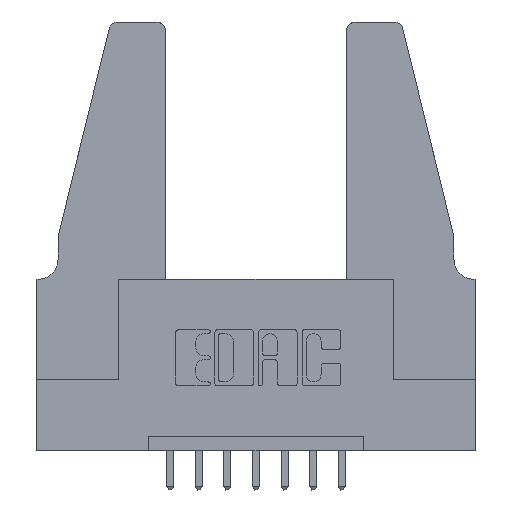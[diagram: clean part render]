
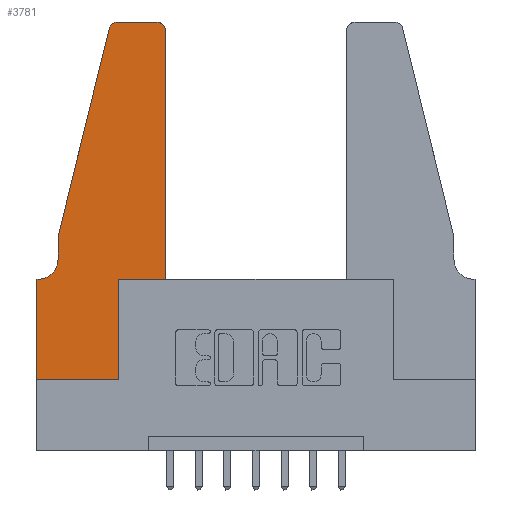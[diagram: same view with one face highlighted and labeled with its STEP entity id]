
A CAD part, top view. The second image highlights one B-rep face of the part: STEP entity #3781.
In plain terms, the highlighted planar face has unit normal (0, 0, 1).
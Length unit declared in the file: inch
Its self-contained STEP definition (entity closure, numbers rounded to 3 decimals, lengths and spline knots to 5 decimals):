
#124 = ORIENTED_EDGE ( 'NONE', *, *, #11380, .T. ) ;
#165 = ORIENTED_EDGE ( 'NONE', *, *, #5843, .T. ) ;
#197 = CARTESIAN_POINT ( 'NONE',  ( 0.4205, 1.25, 0.37 ) ) ;
#277 = VERTEX_POINT ( 'NONE', #3171 ) ;
#298 = VERTEX_POINT ( 'NONE', #10692 ) ;
#717 = CARTESIAN_POINT ( 'NONE',  ( 0., 0., 0.37 ) ) ;
#775 = CARTESIAN_POINT ( 'NONE',  ( 0.284, 1.22, 0.37 ) ) ;
#945 = LINE ( 'NONE', #11992, #2404 ) ;
#967 = VECTOR ( 'NONE', #8117, 39.37008 ) ;
#993 = ORIENTED_EDGE ( 'NONE', *, *, #7801, .T. ) ;
#1168 = VECTOR ( 'NONE', #8905, 39.37008 ) ;
#1172 = ORIENTED_EDGE ( 'NONE', *, *, #2631, .T. ) ;
#1246 = CARTESIAN_POINT ( 'NONE',  ( 0., 0.35, 0.37 ) ) ;
#1318 = LINE ( 'NONE', #10766, #1168 ) ;
#1461 = VECTOR ( 'NONE', #8298, 39.37008 ) ;
#1601 = DIRECTION ( 'NONE',  ( 0., -1., 0. ) ) ;
#1674 = CARTESIAN_POINT ( 'NONE',  ( 0.0755, 0.35, 0.37 ) ) ;
#1725 = VECTOR ( 'NONE', #11046, 39.37008 ) ;
#1729 = ORIENTED_EDGE ( 'NONE', *, *, #4558, .T. ) ;
#1807 = LINE ( 'NONE', #717, #8303 ) ;
#2016 = AXIS2_PLACEMENT_3D ( 'NONE', #775, #5501, #10247 ) ;
#2052 = DIRECTION ( 'NONE',  ( 1., 0., 0. ) ) ;
#2154 = VERTEX_POINT ( 'NONE', #5030 ) ;
#2197 = VERTEX_POINT ( 'NONE', #3082 ) ;
#2404 = VECTOR ( 'NONE', #8338, 39.37008 ) ;
#2524 = DIRECTION ( 'NONE',  ( -1., 0., 0. ) ) ;
#2631 = EDGE_CURVE ( 'NONE', #277, #5910, #1318, .T. ) ;
#2647 = VECTOR ( 'NONE', #7125, 39.37008 ) ;
#2732 = DIRECTION ( 'NONE',  ( 0., 0., -1. ) ) ;
#2892 = AXIS2_PLACEMENT_3D ( 'NONE', #4583, #2732, #11048 ) ;
#3082 = CARTESIAN_POINT ( 'NONE',  ( 0., 0.35, 0.37 ) ) ;
#3114 = DIRECTION ( 'NONE',  ( 0., 0., 1. ) ) ;
#3171 = CARTESIAN_POINT ( 'NONE',  ( 0.0755, 0.5, 0.37 ) ) ;
#3208 = EDGE_CURVE ( 'NONE', #8248, #277, #945, .T. ) ;
#3739 = VERTEX_POINT ( 'NONE', #3897 ) ;
#3781 = ADVANCED_FACE ( 'NONE', ( #11063 ), #6969, .T. ) ;
#3893 = EDGE_CURVE ( 'NONE', #5910, #9543, #11351, .T. ) ;
#3897 = CARTESIAN_POINT ( 'NONE',  ( 0., 0., 0.37 ) ) ;
#3913 = LINE ( 'NONE', #8070, #967 ) ;
#3996 = CARTESIAN_POINT ( 'NONE',  ( 0.4205, 1.22, 0.37 ) ) ;
#4053 = EDGE_CURVE ( 'NONE', #7794, #2154, #8700, .T. ) ;
#4058 = VECTOR ( 'NONE', #2524, 39.37008 ) ;
#4100 = CARTESIAN_POINT ( 'NONE',  ( 0.0055, 0.35, 0.37 ) ) ;
#4126 = EDGE_CURVE ( 'NONE', #3739, #11716, #10029, .T. ) ;
#4273 = CARTESIAN_POINT ( 'NONE',  ( 0.25487, 1.22718, 0.37 ) ) ;
#4558 = EDGE_CURVE ( 'NONE', #8471, #298, #9291, .T. ) ;
#4583 = CARTESIAN_POINT ( 'NONE',  ( 0.0055, 0.42, 0.37 ) ) ;
#4622 = AXIS2_PLACEMENT_3D ( 'NONE', #1246, #6121, #9825 ) ;
#4692 = LINE ( 'NONE', #7117, #1725 ) ;
#4745 = EDGE_CURVE ( 'NONE', #2154, #8471, #5001, .T. ) ;
#4814 = CARTESIAN_POINT ( 'NONE',  ( 0.4505, 0.35, 0.37 ) ) ;
#5001 = CIRCLE ( 'NONE', #10412, 0.03 ) ;
#5030 = CARTESIAN_POINT ( 'NONE',  ( 0.4505, 1.22, 0.37 ) ) ;
#5501 = DIRECTION ( 'NONE',  ( 0., 0., 1. ) ) ;
#5579 = DIRECTION ( 'NONE',  ( 1., 0., 0. ) ) ;
#5729 = ORIENTED_EDGE ( 'NONE', *, *, #9223, .T. ) ;
#5766 = ORIENTED_EDGE ( 'NONE', *, *, #3893, .T. ) ;
#5843 = EDGE_CURVE ( 'NONE', #11716, #9695, #4692, .T. ) ;
#5910 = VERTEX_POINT ( 'NONE', #7242 ) ;
#6121 = DIRECTION ( 'NONE',  ( 0., 0., 1. ) ) ;
#6367 = CARTESIAN_POINT ( 'NONE',  ( 0.4505, 0.35, 0.37 ) ) ;
#6519 = ORIENTED_EDGE ( 'NONE', *, *, #3208, .T. ) ;
#6968 = CARTESIAN_POINT ( 'NONE',  ( 0.2605, 1.25, 0.37 ) ) ;
#6969 = PLANE ( 'NONE',  #4622 ) ;
#7117 = CARTESIAN_POINT ( 'NONE',  ( 0.2865, 0.35, 0.37 ) ) ;
#7125 = DIRECTION ( 'NONE',  ( -1., 0., 0. ) ) ;
#7242 = CARTESIAN_POINT ( 'NONE',  ( 0.0755, 0.42, 0.37 ) ) ;
#7351 = ORIENTED_EDGE ( 'NONE', *, *, #7895, .T. ) ;
#7791 = ORIENTED_EDGE ( 'NONE', *, *, #4126, .T. ) ;
#7794 = VERTEX_POINT ( 'NONE', #4814 ) ;
#7801 = EDGE_CURVE ( 'NONE', #9695, #7794, #3913, .T. ) ;
#7895 = EDGE_CURVE ( 'NONE', #9543, #2197, #9375, .T. ) ;
#7976 = ORIENTED_EDGE ( 'NONE', *, *, #4745, .T. ) ;
#8070 = CARTESIAN_POINT ( 'NONE',  ( 0.4505, 0.35, 0.37 ) ) ;
#8117 = DIRECTION ( 'NONE',  ( 1., 0., 0. ) ) ;
#8248 = VERTEX_POINT ( 'NONE', #4273 ) ;
#8298 = DIRECTION ( 'NONE',  ( 0., 1., 0. ) ) ;
#8303 = VECTOR ( 'NONE', #1601, 39.37008 ) ;
#8338 = DIRECTION ( 'NONE',  ( -0.239, -0.971, 0. ) ) ;
#8471 = VERTEX_POINT ( 'NONE', #197 ) ;
#8602 = CIRCLE ( 'NONE', #2016, 0.03 ) ;
#8700 = LINE ( 'NONE', #6367, #1461 ) ;
#8905 = DIRECTION ( 'NONE',  ( 0., -1., 0. ) ) ;
#9223 = EDGE_CURVE ( 'NONE', #298, #8248, #8602, .T. ) ;
#9253 = ORIENTED_EDGE ( 'NONE', *, *, #4053, .T. ) ;
#9291 = LINE ( 'NONE', #6968, #2647 ) ;
#9375 = LINE ( 'NONE', #1674, #4058 ) ;
#9445 = VECTOR ( 'NONE', #5579, 39.37008 ) ;
#9543 = VERTEX_POINT ( 'NONE', #4100 ) ;
#9695 = VERTEX_POINT ( 'NONE', #11960 ) ;
#9825 = DIRECTION ( 'NONE',  ( 1., 0., 0. ) ) ;
#10029 = LINE ( 'NONE', #11226, #9445 ) ;
#10247 = DIRECTION ( 'NONE',  ( 1., 0., 0. ) ) ;
#10412 = AXIS2_PLACEMENT_3D ( 'NONE', #3996, #3114, #2052 ) ;
#10598 = CARTESIAN_POINT ( 'NONE',  ( 0.2865, 0., 0.37 ) ) ;
#10692 = CARTESIAN_POINT ( 'NONE',  ( 0.284, 1.25, 0.37 ) ) ;
#10766 = CARTESIAN_POINT ( 'NONE',  ( 0.0755, 0.5, 0.37 ) ) ;
#11046 = DIRECTION ( 'NONE',  ( 0., 1., 0. ) ) ;
#11048 = DIRECTION ( 'NONE',  ( -1., 0., 0. ) ) ;
#11063 = FACE_OUTER_BOUND ( 'NONE', #11568, .T. ) ;
#11226 = CARTESIAN_POINT ( 'NONE',  ( 0., 0., 0.37 ) ) ;
#11351 = CIRCLE ( 'NONE', #2892, 0.07 ) ;
#11380 = EDGE_CURVE ( 'NONE', #2197, #3739, #1807, .T. ) ;
#11568 = EDGE_LOOP ( 'NONE', ( #1729, #5729, #6519, #1172, #5766, #7351, #124, #7791, #165, #993, #9253, #7976 ) ) ;
#11716 = VERTEX_POINT ( 'NONE', #10598 ) ;
#11960 = CARTESIAN_POINT ( 'NONE',  ( 0.2865, 0.35, 0.37 ) ) ;
#11992 = CARTESIAN_POINT ( 'NONE',  ( 0.0755, 0.5, 0.37 ) ) ;
